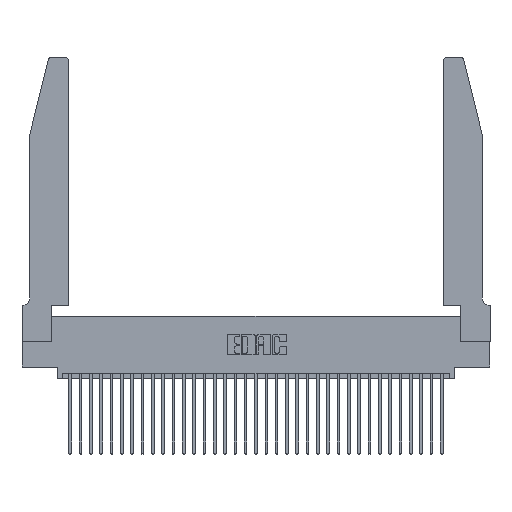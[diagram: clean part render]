
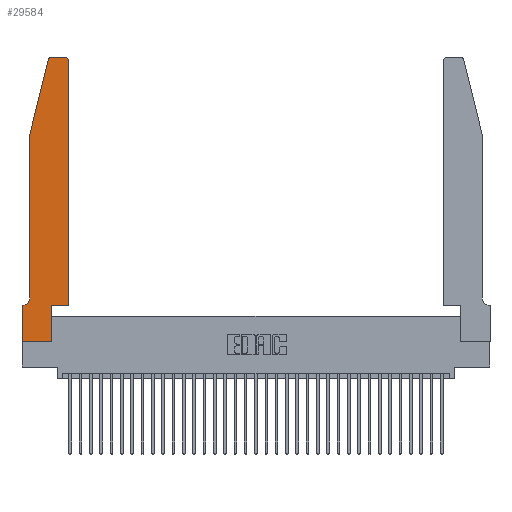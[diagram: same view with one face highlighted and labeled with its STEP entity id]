
A CAD part, top view. The second image highlights one B-rep face of the part: STEP entity #29584.
In plain terms, the highlighted planar face has unit normal (0, 0, 1).
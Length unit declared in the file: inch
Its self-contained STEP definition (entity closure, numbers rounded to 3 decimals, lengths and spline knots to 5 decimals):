
#39 = EDGE_CURVE ( 'NONE', #20644, #7298, #20806, .T. ) ;
#206 = ORIENTED_EDGE ( 'NONE', *, *, #21389, .T. ) ;
#256 = ORIENTED_EDGE ( 'NONE', *, *, #17477, .T. ) ;
#1973 = CARTESIAN_POINT ( 'NONE',  ( 0.0055, 0.42, 0.37 ) ) ;
#2075 = EDGE_CURVE ( 'NONE', #28702, #13959, #17312, .T. ) ;
#2081 = DIRECTION ( 'NONE',  ( 0., 0., 1. ) ) ;
#2975 = EDGE_CURVE ( 'NONE', #13119, #22206, #6334, .T. ) ;
#3291 = ORIENTED_EDGE ( 'NONE', *, *, #13042, .T. ) ;
#3507 = LINE ( 'NONE', #21586, #18992 ) ;
#3731 = VERTEX_POINT ( 'NONE', #6351 ) ;
#3873 = DIRECTION ( 'NONE',  ( 0., -1., 0. ) ) ;
#4232 = LINE ( 'NONE', #29672, #14204 ) ;
#4313 = EDGE_CURVE ( 'NONE', #30386, #32475, #28481, .T. ) ;
#4660 = PLANE ( 'NONE',  #16939 ) ;
#5849 = CARTESIAN_POINT ( 'NONE',  ( 0.2865, 0.35, 0.37 ) ) ;
#5891 = LINE ( 'NONE', #11460, #15944 ) ;
#5960 = VECTOR ( 'NONE', #9550, 39.37008 ) ;
#6253 = DIRECTION ( 'NONE',  ( 1., 0., 0. ) ) ;
#6334 = LINE ( 'NONE', #26422, #19672 ) ;
#6351 = CARTESIAN_POINT ( 'NONE',  ( 0.4505, 2.72, 0.37 ) ) ;
#6381 = DIRECTION ( 'NONE',  ( 0., 0., 1. ) ) ;
#6651 = ORIENTED_EDGE ( 'NONE', *, *, #4313, .T. ) ;
#6717 = EDGE_CURVE ( 'NONE', #22206, #30386, #19435, .T. ) ;
#6909 = CARTESIAN_POINT ( 'NONE',  ( 0.4505, 0.35, 0.37 ) ) ;
#7298 = VERTEX_POINT ( 'NONE', #6909 ) ;
#7885 = CARTESIAN_POINT ( 'NONE',  ( 0.2865, 0., 0.37 ) ) ;
#8412 = CARTESIAN_POINT ( 'NONE',  ( 0.25487, 2.72718, 0.37 ) ) ;
#8634 = DIRECTION ( 'NONE',  ( 0., 0., 1. ) ) ;
#8972 = CIRCLE ( 'NONE', #19343, 0.07 ) ;
#9158 = CARTESIAN_POINT ( 'NONE',  ( 0.4205, 2.72, 0.37 ) ) ;
#9422 = AXIS2_PLACEMENT_3D ( 'NONE', #21948, #8634, #27352 ) ;
#9550 = DIRECTION ( 'NONE',  ( 0., 1., 0. ) ) ;
#9905 = VERTEX_POINT ( 'NONE', #26621 ) ;
#10036 = DIRECTION ( 'NONE',  ( 0., 0., -1. ) ) ;
#10156 = DIRECTION ( 'NONE',  ( -1., 0., 0. ) ) ;
#10410 = DIRECTION ( 'NONE',  ( -1., 0., 0. ) ) ;
#10480 = CARTESIAN_POINT ( 'NONE',  ( 0.4205, 2.75, 0.37 ) ) ;
#10618 = DIRECTION ( 'NONE',  ( -1., 0., 0. ) ) ;
#10643 = CARTESIAN_POINT ( 'NONE',  ( 0.4505, 0.35, 0.37 ) ) ;
#10776 = DIRECTION ( 'NONE',  ( 1., 0., 0. ) ) ;
#11003 = VECTOR ( 'NONE', #10776, 39.37008 ) ;
#11460 = CARTESIAN_POINT ( 'NONE',  ( 0., 0., 0.37 ) ) ;
#12195 = ORIENTED_EDGE ( 'NONE', *, *, #25536, .T. ) ;
#12335 = CARTESIAN_POINT ( 'NONE',  ( 0.2865, 0.35, 0.37 ) ) ;
#12596 = CARTESIAN_POINT ( 'NONE',  ( 0., 0.35, 0.37 ) ) ;
#12800 = LINE ( 'NONE', #10643, #25748 ) ;
#13042 = EDGE_CURVE ( 'NONE', #9905, #34388, #8972, .T. ) ;
#13119 = VERTEX_POINT ( 'NONE', #10480 ) ;
#13436 = DIRECTION ( 'NONE',  ( 0., 1., 0. ) ) ;
#13658 = VECTOR ( 'NONE', #34051, 39.37008 ) ;
#13959 = VERTEX_POINT ( 'NONE', #7885 ) ;
#14085 = CARTESIAN_POINT ( 'NONE',  ( 0.0755, 2., 0.37 ) ) ;
#14204 = VECTOR ( 'NONE', #10618, 39.37008 ) ;
#15104 = FACE_OUTER_BOUND ( 'NONE', #16004, .T. ) ;
#15484 = CARTESIAN_POINT ( 'NONE',  ( 0., 0.35, 0.37 ) ) ;
#15944 = VECTOR ( 'NONE', #3873, 39.37008 ) ;
#16004 = EDGE_LOOP ( 'NONE', ( #28577, #20960, #6651, #24074, #3291, #12195, #256, #33178, #17542, #18021, #206, #29198 ) ) ;
#16704 = CARTESIAN_POINT ( 'NONE',  ( 0., 0., 0.37 ) ) ;
#16939 = AXIS2_PLACEMENT_3D ( 'NONE', #12596, #2081, #23221 ) ;
#17312 = LINE ( 'NONE', #18708, #11003 ) ;
#17477 = EDGE_CURVE ( 'NONE', #23533, #28702, #5891, .T. ) ;
#17542 = ORIENTED_EDGE ( 'NONE', *, *, #24609, .T. ) ;
#17586 = VECTOR ( 'NONE', #24816, 39.37008 ) ;
#18021 = ORIENTED_EDGE ( 'NONE', *, *, #39, .T. ) ;
#18584 = EDGE_CURVE ( 'NONE', #3731, #13119, #21302, .T. ) ;
#18708 = CARTESIAN_POINT ( 'NONE',  ( 0., 0., 0.37 ) ) ;
#18992 = VECTOR ( 'NONE', #32595, 39.37008 ) ;
#19118 = CARTESIAN_POINT ( 'NONE',  ( 0.0755, 2., 0.37 ) ) ;
#19343 = AXIS2_PLACEMENT_3D ( 'NONE', #1973, #10036, #10156 ) ;
#19435 = CIRCLE ( 'NONE', #9422, 0.03 ) ;
#19672 = VECTOR ( 'NONE', #10410, 39.37008 ) ;
#20644 = VERTEX_POINT ( 'NONE', #5849 ) ;
#20806 = LINE ( 'NONE', #27116, #13658 ) ;
#20960 = ORIENTED_EDGE ( 'NONE', *, *, #6717, .T. ) ;
#21302 = CIRCLE ( 'NONE', #34526, 0.03 ) ;
#21389 = EDGE_CURVE ( 'NONE', #7298, #3731, #12800, .T. ) ;
#21586 = CARTESIAN_POINT ( 'NONE',  ( 0.0755, 2., 0.37 ) ) ;
#21948 = CARTESIAN_POINT ( 'NONE',  ( 0.284, 2.72, 0.37 ) ) ;
#22206 = VERTEX_POINT ( 'NONE', #23042 ) ;
#22222 = CARTESIAN_POINT ( 'NONE',  ( 0.0055, 0.35, 0.37 ) ) ;
#23042 = CARTESIAN_POINT ( 'NONE',  ( 0.284, 2.75, 0.37 ) ) ;
#23221 = DIRECTION ( 'NONE',  ( 1., 0., 0. ) ) ;
#23533 = VERTEX_POINT ( 'NONE', #15484 ) ;
#24074 = ORIENTED_EDGE ( 'NONE', *, *, #32912, .T. ) ;
#24609 = EDGE_CURVE ( 'NONE', #13959, #20644, #27281, .T. ) ;
#24816 = DIRECTION ( 'NONE',  ( -0.239, -0.971, 0. ) ) ;
#25536 = EDGE_CURVE ( 'NONE', #34388, #23533, #4232, .T. ) ;
#25748 = VECTOR ( 'NONE', #13436, 39.37008 ) ;
#26422 = CARTESIAN_POINT ( 'NONE',  ( 0.2605, 2.75, 0.37 ) ) ;
#26621 = CARTESIAN_POINT ( 'NONE',  ( 0.0755, 0.42, 0.37 ) ) ;
#27116 = CARTESIAN_POINT ( 'NONE',  ( 0.4505, 0.35, 0.37 ) ) ;
#27281 = LINE ( 'NONE', #12335, #5960 ) ;
#27352 = DIRECTION ( 'NONE',  ( 1., 0., 0. ) ) ;
#28481 = LINE ( 'NONE', #14085, #17586 ) ;
#28577 = ORIENTED_EDGE ( 'NONE', *, *, #2975, .T. ) ;
#28702 = VERTEX_POINT ( 'NONE', #16704 ) ;
#29198 = ORIENTED_EDGE ( 'NONE', *, *, #18584, .T. ) ;
#29584 = ADVANCED_FACE ( 'NONE', ( #15104 ), #4660, .T. ) ;
#29672 = CARTESIAN_POINT ( 'NONE',  ( 0.0755, 0.35, 0.37 ) ) ;
#30386 = VERTEX_POINT ( 'NONE', #8412 ) ;
#32475 = VERTEX_POINT ( 'NONE', #19118 ) ;
#32595 = DIRECTION ( 'NONE',  ( 0., -1., 0. ) ) ;
#32912 = EDGE_CURVE ( 'NONE', #32475, #9905, #3507, .T. ) ;
#33178 = ORIENTED_EDGE ( 'NONE', *, *, #2075, .T. ) ;
#34051 = DIRECTION ( 'NONE',  ( 1., 0., 0. ) ) ;
#34388 = VERTEX_POINT ( 'NONE', #22222 ) ;
#34526 = AXIS2_PLACEMENT_3D ( 'NONE', #9158, #6381, #6253 ) ;
